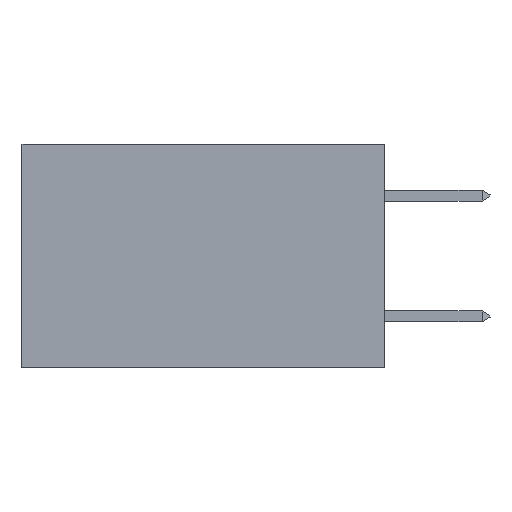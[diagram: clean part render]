
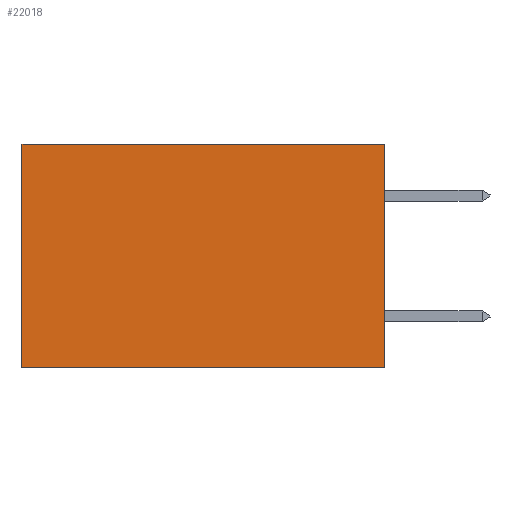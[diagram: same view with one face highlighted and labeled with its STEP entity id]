
A CAD part, left-side view. The second image highlights one B-rep face of the part: STEP entity #22018.
In plain terms, the highlighted planar face has unit normal (-1, 0, 0).
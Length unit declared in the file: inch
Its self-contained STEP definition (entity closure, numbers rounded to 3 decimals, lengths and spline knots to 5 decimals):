
#852 = CARTESIAN_POINT ( 'NONE',  ( 0.2875, 0.6, 0. ) ) ;
#1018 = DIRECTION ( 'NONE',  ( 0., 0., -1. ) ) ;
#2565 = PLANE ( 'NONE',  #6107 ) ;
#2584 = ORIENTED_EDGE ( 'NONE', *, *, #31205, .F. ) ;
#3423 = EDGE_CURVE ( 'NONE', #20169, #15424, #11266, .T. ) ;
#3851 = VECTOR ( 'NONE', #1018, 39.37008 ) ;
#6107 = AXIS2_PLACEMENT_3D ( 'NONE', #13782, #32619, #16477 ) ;
#7883 = LINE ( 'NONE', #10801, #22260 ) ;
#8059 = VERTEX_POINT ( 'NONE', #24969 ) ;
#9027 = CARTESIAN_POINT ( 'NONE',  ( 0.2875, 0., -0.37 ) ) ;
#9134 = CARTESIAN_POINT ( 'NONE',  ( 0.2875, 0., 0. ) ) ;
#10801 = CARTESIAN_POINT ( 'NONE',  ( 0.2875, 0., -0.37 ) ) ;
#10923 = DIRECTION ( 'NONE',  ( 0., 1., 0. ) ) ;
#11254 = CARTESIAN_POINT ( 'NONE',  ( 0.2875, 0.6, -0.37 ) ) ;
#11266 = LINE ( 'NONE', #852, #3851 ) ;
#12373 = DIRECTION ( 'NONE',  ( 0., 0., -1. ) ) ;
#13495 = EDGE_CURVE ( 'NONE', #8059, #20169, #33691, .T. ) ;
#13782 = CARTESIAN_POINT ( 'NONE',  ( 0.2875, 0., 0. ) ) ;
#14191 = ORIENTED_EDGE ( 'NONE', *, *, #13495, .T. ) ;
#15424 = VERTEX_POINT ( 'NONE', #11254 ) ;
#16477 = DIRECTION ( 'NONE',  ( 0., 0., -1. ) ) ;
#19752 = VECTOR ( 'NONE', #12373, 39.37008 ) ;
#19855 = EDGE_CURVE ( 'NONE', #26839, #15424, #7883, .T. ) ;
#20169 = VERTEX_POINT ( 'NONE', #33563 ) ;
#22018 = ADVANCED_FACE ( 'NONE', ( #22094 ), #2565, .F. ) ;
#22094 = FACE_OUTER_BOUND ( 'NONE', #25839, .T. ) ;
#22260 = VECTOR ( 'NONE', #10923, 39.37008 ) ;
#24969 = CARTESIAN_POINT ( 'NONE',  ( 0.2875, 0., 0. ) ) ;
#25839 = EDGE_LOOP ( 'NONE', ( #30272, #31239, #2584, #14191 ) ) ;
#26839 = VERTEX_POINT ( 'NONE', #9027 ) ;
#28039 = DIRECTION ( 'NONE',  ( 0., 1., 0. ) ) ;
#30272 = ORIENTED_EDGE ( 'NONE', *, *, #3423, .T. ) ;
#31205 = EDGE_CURVE ( 'NONE', #8059, #26839, #33268, .T. ) ;
#31216 = CARTESIAN_POINT ( 'NONE',  ( 0.2875, 0., 0. ) ) ;
#31239 = ORIENTED_EDGE ( 'NONE', *, *, #19855, .F. ) ;
#32619 = DIRECTION ( 'NONE',  ( 1., 0., 0. ) ) ;
#33268 = LINE ( 'NONE', #31216, #19752 ) ;
#33563 = CARTESIAN_POINT ( 'NONE',  ( 0.2875, 0.6, 0. ) ) ;
#33691 = LINE ( 'NONE', #9134, #34517 ) ;
#34517 = VECTOR ( 'NONE', #28039, 39.37008 ) ;
